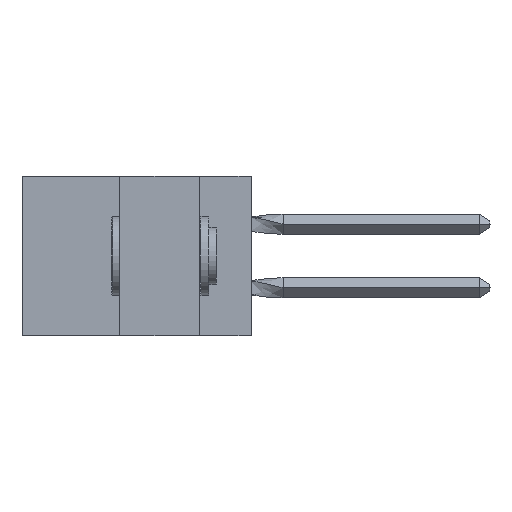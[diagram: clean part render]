
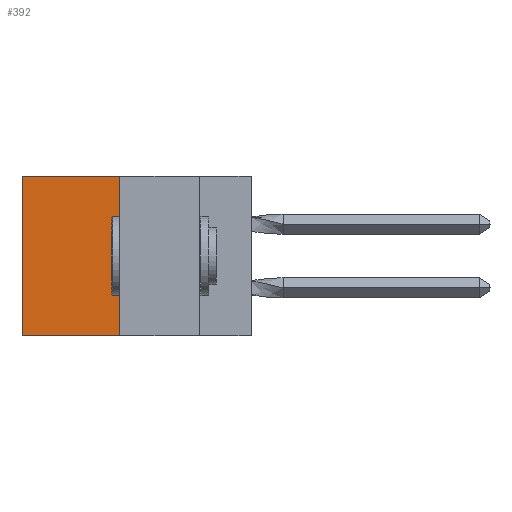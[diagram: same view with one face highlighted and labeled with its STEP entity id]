
A CAD part, left-side view. The second image highlights one B-rep face of the part: STEP entity #392.
In plain terms, the highlighted planar face has unit normal (-1, 0, 0).
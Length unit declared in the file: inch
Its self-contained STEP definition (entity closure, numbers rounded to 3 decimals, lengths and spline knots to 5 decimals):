
#46 = CARTESIAN_POINT ( 'NONE',  ( 0.305, 0.413, 0. ) ) ;
#392 = ADVANCED_FACE ( 'NONE', ( #17277 ), #1110, .F. ) ;
#1001 = EDGE_CURVE ( 'NONE', #20019, #22225, #16372, .T. ) ;
#1038 = CARTESIAN_POINT ( 'NONE',  ( 0.305, 0.413, -0.5 ) ) ;
#1110 = PLANE ( 'NONE',  #19997 ) ;
#1199 = DIRECTION ( 'NONE',  ( 1., 0., 0. ) ) ;
#2845 = DIRECTION ( 'NONE',  ( 0., 1., 0. ) ) ;
#3394 = CARTESIAN_POINT ( 'NONE',  ( 0.305, 0.72, 0. ) ) ;
#6132 = ORIENTED_EDGE ( 'NONE', *, *, #1001, .T. ) ;
#7198 = EDGE_CURVE ( 'NONE', #12601, #20019, #12504, .T. ) ;
#8308 = CARTESIAN_POINT ( 'NONE',  ( 0.305, 0.72, -0.5 ) ) ;
#8420 = DIRECTION ( 'NONE',  ( 0., 0., -1. ) ) ;
#9478 = VERTEX_POINT ( 'NONE', #22247 ) ;
#11549 = EDGE_CURVE ( 'NONE', #9478, #22225, #20090, .T. ) ;
#12424 = EDGE_LOOP ( 'NONE', ( #6132, #22757, #16781, #22243 ) ) ;
#12504 = LINE ( 'NONE', #15454, #20587 ) ;
#12601 = VERTEX_POINT ( 'NONE', #46 ) ;
#13011 = VECTOR ( 'NONE', #23550, 39.37008 ) ;
#15199 = VECTOR ( 'NONE', #22514, 39.37008 ) ;
#15454 = CARTESIAN_POINT ( 'NONE',  ( 0.305, 0.413, 0. ) ) ;
#16372 = LINE ( 'NONE', #8308, #18121 ) ;
#16781 = ORIENTED_EDGE ( 'NONE', *, *, #16841, .F. ) ;
#16841 = EDGE_CURVE ( 'NONE', #12601, #9478, #17084, .T. ) ;
#17084 = LINE ( 'NONE', #19711, #13011 ) ;
#17277 = FACE_OUTER_BOUND ( 'NONE', #12424, .T. ) ;
#18121 = VECTOR ( 'NONE', #21257, 39.37008 ) ;
#19711 = CARTESIAN_POINT ( 'NONE',  ( 0.305, 0.413, -0.5 ) ) ;
#19821 = CARTESIAN_POINT ( 'NONE',  ( 0.305, 0.72, -0.5 ) ) ;
#19997 = AXIS2_PLACEMENT_3D ( 'NONE', #1038, #1199, #8420 ) ;
#20019 = VERTEX_POINT ( 'NONE', #3394 ) ;
#20090 = LINE ( 'NONE', #22605, #15199 ) ;
#20587 = VECTOR ( 'NONE', #2845, 39.37008 ) ;
#21257 = DIRECTION ( 'NONE',  ( 0., 0., -1. ) ) ;
#22225 = VERTEX_POINT ( 'NONE', #19821 ) ;
#22243 = ORIENTED_EDGE ( 'NONE', *, *, #7198, .T. ) ;
#22247 = CARTESIAN_POINT ( 'NONE',  ( 0.305, 0.413, -0.5 ) ) ;
#22514 = DIRECTION ( 'NONE',  ( 0., 1., 0. ) ) ;
#22605 = CARTESIAN_POINT ( 'NONE',  ( 0.305, 0.413, -0.5 ) ) ;
#22757 = ORIENTED_EDGE ( 'NONE', *, *, #11549, .F. ) ;
#23550 = DIRECTION ( 'NONE',  ( 0., 0., -1. ) ) ;
